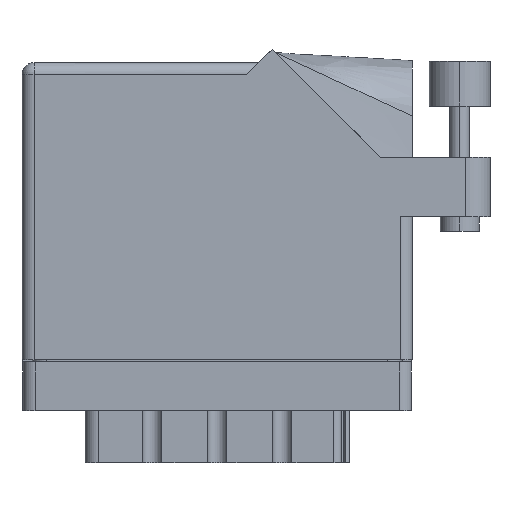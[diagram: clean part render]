
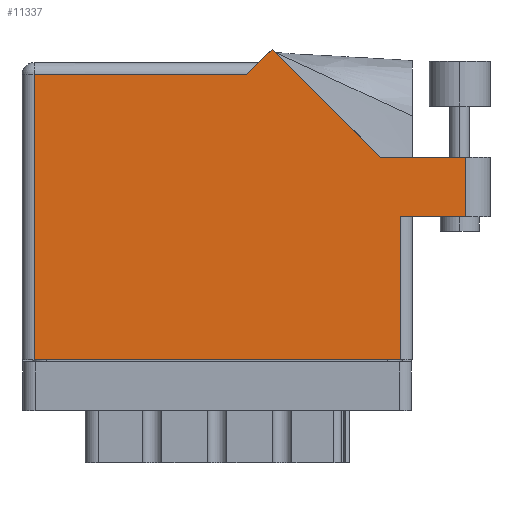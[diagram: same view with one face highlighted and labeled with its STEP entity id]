
A CAD part, front view. The second image highlights one B-rep face of the part: STEP entity #11337.
In plain terms, the highlighted face is planar.
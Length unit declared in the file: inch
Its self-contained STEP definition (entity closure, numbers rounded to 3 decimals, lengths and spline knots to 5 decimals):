
#499 = LINE ( 'NONE', #25715, #4090 ) ;
#1061 = DIRECTION ( 'NONE',  ( 0., 0., -1. ) ) ;
#1094 = LINE ( 'NONE', #37178, #36086 ) ;
#1443 = EDGE_CURVE ( 'NONE', #25143, #35604, #499, .T. ) ;
#1763 = EDGE_CURVE ( 'NONE', #28696, #2689, #25087, .T. ) ;
#2201 = CARTESIAN_POINT ( 'NONE',  ( 1.948, 0.737, 0. ) ) ;
#2491 = ORIENTED_EDGE ( 'NONE', *, *, #16476, .T. ) ;
#2689 = VERTEX_POINT ( 'NONE', #2201 ) ;
#3782 = CARTESIAN_POINT ( 'NONE',  ( 2.01, 0.737, 0. ) ) ;
#3959 = DIRECTION ( 'NONE',  ( -1., 0., 0. ) ) ;
#4090 = VECTOR ( 'NONE', #34784, 39.37008 ) ;
#6257 = EDGE_CURVE ( 'NONE', #29037, #28696, #1094, .T. ) ;
#6599 = PLANE ( 'NONE',  #36583 ) ;
#6660 = DIRECTION ( 'NONE',  ( 1., 0., 0. ) ) ;
#6720 = CARTESIAN_POINT ( 'NONE',  ( 0., 1.53, 0. ) ) ;
#7617 = ORIENTED_EDGE ( 'NONE', *, *, #1763, .T. ) ;
#7839 = EDGE_CURVE ( 'NONE', #16089, #25143, #26527, .T. ) ;
#8090 = VERTEX_POINT ( 'NONE', #12563 ) ;
#9235 = DIRECTION ( 'NONE',  ( -0.707, -0.707, 0. ) ) ;
#9775 = VECTOR ( 'NONE', #10562, 39.37008 ) ;
#9827 = LINE ( 'NONE', #26332, #18756 ) ;
#10190 = CARTESIAN_POINT ( 'NONE',  ( 0., 1.468, 0. ) ) ;
#10498 = CARTESIAN_POINT ( 'NONE',  ( 2.285, 0.737, 0. ) ) ;
#10562 = DIRECTION ( 'NONE',  ( -0.707, 0.707, 0. ) ) ;
#10658 = VERTEX_POINT ( 'NONE', #24173 ) ;
#11337 = ADVANCED_FACE ( 'NONE', ( #20867 ), #6599, .F. ) ;
#11415 = ORIENTED_EDGE ( 'NONE', *, *, #7839, .T. ) ;
#11454 = CARTESIAN_POINT ( 'NONE',  ( 2.285, 1.044, 0. ) ) ;
#11678 = ORIENTED_EDGE ( 'NONE', *, *, #6257, .T. ) ;
#12066 = VERTEX_POINT ( 'NONE', #13097 ) ;
#12563 = CARTESIAN_POINT ( 'NONE',  ( 1.28771, 1.60071, 0. ) ) ;
#13097 = CARTESIAN_POINT ( 'NONE',  ( 1.155, 1.468, 0. ) ) ;
#13284 = VECTOR ( 'NONE', #24448, 39.37008 ) ;
#13586 = ORIENTED_EDGE ( 'NONE', *, *, #1443, .T. ) ;
#14400 = VECTOR ( 'NONE', #31513, 39.37008 ) ;
#14791 = CARTESIAN_POINT ( 'NONE',  ( 0.062, 0., 0. ) ) ;
#15313 = EDGE_CURVE ( 'NONE', #10658, #29037, #9827, .T. ) ;
#16089 = VERTEX_POINT ( 'NONE', #10498 ) ;
#16138 = CARTESIAN_POINT ( 'NONE',  ( 1.948, 0.737, 0. ) ) ;
#16476 = EDGE_CURVE ( 'NONE', #8090, #12066, #25351, .T. ) ;
#16557 = VECTOR ( 'NONE', #21897, 39.37008 ) ;
#17679 = DIRECTION ( 'NONE',  ( 0., -1., 0. ) ) ;
#17904 = ORIENTED_EDGE ( 'NONE', *, *, #34698, .T. ) ;
#18708 = ORIENTED_EDGE ( 'NONE', *, *, #15313, .T. ) ;
#18756 = VECTOR ( 'NONE', #17679, 39.37008 ) ;
#19387 = CARTESIAN_POINT ( 'NONE',  ( 1.84442, 1.044, 0. ) ) ;
#19741 = DIRECTION ( 'NONE',  ( 1., 0., 0. ) ) ;
#20867 = FACE_OUTER_BOUND ( 'NONE', #23850, .T. ) ;
#21897 = DIRECTION ( 'NONE',  ( 0., 1., 0. ) ) ;
#23564 = LINE ( 'NONE', #3782, #29414 ) ;
#23850 = EDGE_LOOP ( 'NONE', ( #31275, #11415, #13586, #31177, #2491, #17904, #18708, #11678, #7617 ) ) ;
#24018 = CARTESIAN_POINT ( 'NONE',  ( 2.285, 1.044, 0. ) ) ;
#24173 = CARTESIAN_POINT ( 'NONE',  ( 0.062, 1.468, 0. ) ) ;
#24448 = DIRECTION ( 'NONE',  ( -1., 0., 0. ) ) ;
#25074 = CARTESIAN_POINT ( 'NONE',  ( 1.84442, 1.044, 0. ) ) ;
#25087 = LINE ( 'NONE', #16138, #16557 ) ;
#25143 = VERTEX_POINT ( 'NONE', #24018 ) ;
#25351 = LINE ( 'NONE', #26874, #29391 ) ;
#25715 = CARTESIAN_POINT ( 'NONE',  ( 2.41, 1.044, 0. ) ) ;
#26332 = CARTESIAN_POINT ( 'NONE',  ( 0.062, 0., 0. ) ) ;
#26527 = LINE ( 'NONE', #11454, #14400 ) ;
#26874 = CARTESIAN_POINT ( 'NONE',  ( 1.217, 1.53, 0. ) ) ;
#28602 = EDGE_CURVE ( 'NONE', #35604, #8090, #31708, .T. ) ;
#28696 = VERTEX_POINT ( 'NONE', #30970 ) ;
#29037 = VERTEX_POINT ( 'NONE', #14791 ) ;
#29391 = VECTOR ( 'NONE', #9235, 39.37008 ) ;
#29414 = VECTOR ( 'NONE', #6660, 39.37008 ) ;
#30970 = CARTESIAN_POINT ( 'NONE',  ( 1.948, 0., 0. ) ) ;
#31177 = ORIENTED_EDGE ( 'NONE', *, *, #28602, .T. ) ;
#31275 = ORIENTED_EDGE ( 'NONE', *, *, #35187, .T. ) ;
#31513 = DIRECTION ( 'NONE',  ( 0., 1., 0. ) ) ;
#31708 = LINE ( 'NONE', #25074, #9775 ) ;
#34698 = EDGE_CURVE ( 'NONE', #12066, #10658, #35277, .T. ) ;
#34784 = DIRECTION ( 'NONE',  ( -1., 0., 0. ) ) ;
#35187 = EDGE_CURVE ( 'NONE', #2689, #16089, #23564, .T. ) ;
#35277 = LINE ( 'NONE', #10190, #13284 ) ;
#35604 = VERTEX_POINT ( 'NONE', #19387 ) ;
#36086 = VECTOR ( 'NONE', #19741, 39.37008 ) ;
#36583 = AXIS2_PLACEMENT_3D ( 'NONE', #6720, #1061, #3959 ) ;
#37178 = CARTESIAN_POINT ( 'NONE',  ( 0., 0., 0. ) ) ;
